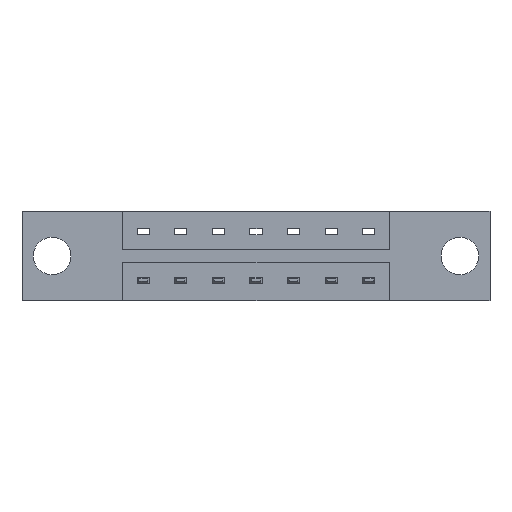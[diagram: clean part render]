
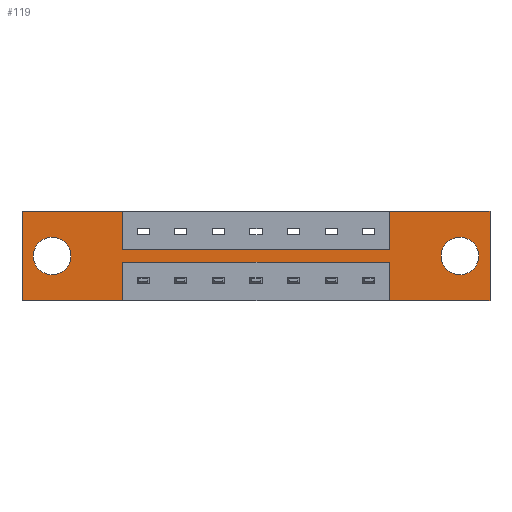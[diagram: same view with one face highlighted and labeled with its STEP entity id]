
A CAD part, front view. The second image highlights one B-rep face of the part: STEP entity #119.
In plain terms, the highlighted planar face has unit normal (0, -1, 0).
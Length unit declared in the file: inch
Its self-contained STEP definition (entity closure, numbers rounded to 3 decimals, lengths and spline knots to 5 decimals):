
#56 = EDGE_CURVE ( 'NONE', #5576, #5710, #2943, .T. ) ;
#72 = AXIS2_PLACEMENT_3D ( 'NONE', #1393, #3893, #1264 ) ;
#119 = ADVANCED_FACE ( 'NONE', ( #5658, #4258, #1630 ), #8319, .T. ) ;
#120 = EDGE_CURVE ( 'NONE', #6968, #8286, #5614, .T. ) ;
#171 = ORIENTED_EDGE ( 'NONE', *, *, #4753, .F. ) ;
#228 = LINE ( 'NONE', #2906, #4995 ) ;
#235 = ORIENTED_EDGE ( 'NONE', *, *, #6564, .F. ) ;
#274 = LINE ( 'NONE', #7508, #5452 ) ;
#319 = VERTEX_POINT ( 'NONE', #5963 ) ;
#415 = LINE ( 'NONE', #5751, #2326 ) ;
#420 = ORIENTED_EDGE ( 'NONE', *, *, #2875, .F. ) ;
#724 = CARTESIAN_POINT ( 'NONE',  ( 0.125, 0., -0.185 ) ) ;
#770 = ORIENTED_EDGE ( 'NONE', *, *, #2677, .F. ) ;
#819 = ORIENTED_EDGE ( 'NONE', *, *, #1943, .F. ) ;
#827 = ORIENTED_EDGE ( 'NONE', *, *, #1180, .F. ) ;
#941 = LINE ( 'NONE', #3728, #6771 ) ;
#965 = VERTEX_POINT ( 'NONE', #3575 ) ;
#981 = CARTESIAN_POINT ( 'NONE',  ( 0.4175, 0., -0.1585 ) ) ;
#1003 = VERTEX_POINT ( 'NONE', #1655 ) ;
#1050 = DIRECTION ( 'NONE',  ( 0., 0., -1. ) ) ;
#1118 = CARTESIAN_POINT ( 'NONE',  ( 0.4175, 0., -0.2115 ) ) ;
#1180 = EDGE_CURVE ( 'NONE', #1003, #2421, #8031, .T. ) ;
#1247 = DIRECTION ( 'NONE',  ( 1., 0., 0. ) ) ;
#1264 = DIRECTION ( 'NONE',  ( 0., 0., 1. ) ) ;
#1393 = CARTESIAN_POINT ( 'NONE',  ( 0.125, 0., -0.185 ) ) ;
#1422 = EDGE_CURVE ( 'NONE', #965, #4962, #941, .T. ) ;
#1538 = CARTESIAN_POINT ( 'NONE',  ( 0., 0., -0.37 ) ) ;
#1548 = VECTOR ( 'NONE', #3085, 39.37008 ) ;
#1630 = FACE_OUTER_BOUND ( 'NONE', #1774, .T. ) ;
#1648 = CARTESIAN_POINT ( 'NONE',  ( 0.4175, 0., -0.2115 ) ) ;
#1655 = CARTESIAN_POINT ( 'NONE',  ( 0., 0., 0. ) ) ;
#1774 = EDGE_LOOP ( 'NONE', ( #2347, #4719, #420, #2455, #770, #3944, #171, #827, #235, #4479, #4236, #819 ) ) ;
#1817 = DIRECTION ( 'NONE',  ( -1., 0., 0. ) ) ;
#1943 = EDGE_CURVE ( 'NONE', #4962, #7129, #228, .T. ) ;
#2043 = VERTEX_POINT ( 'NONE', #3120 ) ;
#2137 = EDGE_CURVE ( 'NONE', #2043, #2488, #8067, .T. ) ;
#2326 = VECTOR ( 'NONE', #3871, 39.37008 ) ;
#2347 = ORIENTED_EDGE ( 'NONE', *, *, #1422, .F. ) ;
#2374 = DIRECTION ( 'NONE',  ( 0., 0., 1. ) ) ;
#2390 = DIRECTION ( 'NONE',  ( 0., 0., -1. ) ) ;
#2394 = VERTEX_POINT ( 'NONE', #3150 ) ;
#2421 = VERTEX_POINT ( 'NONE', #3197 ) ;
#2455 = ORIENTED_EDGE ( 'NONE', *, *, #2630, .F. ) ;
#2488 = VERTEX_POINT ( 'NONE', #2498 ) ;
#2491 = LINE ( 'NONE', #1648, #8175 ) ;
#2498 = CARTESIAN_POINT ( 'NONE',  ( 1.815, 0., -0.263 ) ) ;
#2586 = CIRCLE ( 'NONE', #3675, 0.078 ) ;
#2630 = EDGE_CURVE ( 'NONE', #8416, #3316, #6665, .T. ) ;
#2677 = EDGE_CURVE ( 'NONE', #8286, #8416, #4085, .T. ) ;
#2875 = EDGE_CURVE ( 'NONE', #3316, #319, #274, .T. ) ;
#2906 = CARTESIAN_POINT ( 'NONE',  ( 0.4175, 0., -0.2115 ) ) ;
#2943 = CIRCLE ( 'NONE', #7828, 0.078 ) ;
#3085 = DIRECTION ( 'NONE',  ( 1., 0., 0. ) ) ;
#3120 = CARTESIAN_POINT ( 'NONE',  ( 1.815, 0., -0.107 ) ) ;
#3150 = CARTESIAN_POINT ( 'NONE',  ( 0.4175, 0., -0.37 ) ) ;
#3197 = CARTESIAN_POINT ( 'NONE',  ( 0.4175, 0., 0. ) ) ;
#3316 = VERTEX_POINT ( 'NONE', #3619 ) ;
#3478 = DIRECTION ( 'NONE',  ( 0., 1., 0. ) ) ;
#3533 = DIRECTION ( 'NONE',  ( 0., 0., -1. ) ) ;
#3575 = CARTESIAN_POINT ( 'NONE',  ( 1.5225, 0., -0.37 ) ) ;
#3594 = VECTOR ( 'NONE', #6621, 39.37008 ) ;
#3619 = CARTESIAN_POINT ( 'NONE',  ( 1.94, 0., 0. ) ) ;
#3675 = AXIS2_PLACEMENT_3D ( 'NONE', #7534, #5475, #3533 ) ;
#3728 = CARTESIAN_POINT ( 'NONE',  ( 1.5225, 0., -0.2115 ) ) ;
#3871 = DIRECTION ( 'NONE',  ( 0., 0., 1. ) ) ;
#3874 = AXIS2_PLACEMENT_3D ( 'NONE', #4076, #6699, #6826 ) ;
#3893 = DIRECTION ( 'NONE',  ( 0., 1., 0. ) ) ;
#3944 = ORIENTED_EDGE ( 'NONE', *, *, #120, .F. ) ;
#4076 = CARTESIAN_POINT ( 'NONE',  ( 1.815, 0., -0.185 ) ) ;
#4085 = LINE ( 'NONE', #6580, #3594 ) ;
#4092 = CARTESIAN_POINT ( 'NONE',  ( 0., 0., 0. ) ) ;
#4102 = EDGE_CURVE ( 'NONE', #2394, #4304, #7671, .T. ) ;
#4175 = DIRECTION ( 'NONE',  ( 0., 0., -1. ) ) ;
#4236 = ORIENTED_EDGE ( 'NONE', *, *, #5077, .F. ) ;
#4251 = DIRECTION ( 'NONE',  ( -1., 0., 0. ) ) ;
#4258 = FACE_BOUND ( 'NONE', #6367, .T. ) ;
#4304 = VERTEX_POINT ( 'NONE', #4520 ) ;
#4370 = CARTESIAN_POINT ( 'NONE',  ( 0.4175, 0., -0.1585 ) ) ;
#4452 = VECTOR ( 'NONE', #4251, 39.37008 ) ;
#4479 = ORIENTED_EDGE ( 'NONE', *, *, #4102, .F. ) ;
#4520 = CARTESIAN_POINT ( 'NONE',  ( 0., 0., -0.37 ) ) ;
#4583 = CARTESIAN_POINT ( 'NONE',  ( 0., 0., -0.37 ) ) ;
#4719 = ORIENTED_EDGE ( 'NONE', *, *, #7145, .F. ) ;
#4753 = EDGE_CURVE ( 'NONE', #2421, #6968, #8431, .T. ) ;
#4870 = EDGE_CURVE ( 'NONE', #5710, #5576, #5805, .T. ) ;
#4927 = ORIENTED_EDGE ( 'NONE', *, *, #56, .T. ) ;
#4962 = VERTEX_POINT ( 'NONE', #6770 ) ;
#4995 = VECTOR ( 'NONE', #5572, 39.37008 ) ;
#5077 = EDGE_CURVE ( 'NONE', #7129, #2394, #2491, .T. ) ;
#5161 = CARTESIAN_POINT ( 'NONE',  ( 1.5225, 0., 0. ) ) ;
#5278 = CARTESIAN_POINT ( 'NONE',  ( 0., 0., 0. ) ) ;
#5452 = VECTOR ( 'NONE', #4175, 39.37008 ) ;
#5475 = DIRECTION ( 'NONE',  ( 0., 1., 0. ) ) ;
#5572 = DIRECTION ( 'NONE',  ( -1., 0., 0. ) ) ;
#5576 = VERTEX_POINT ( 'NONE', #7681 ) ;
#5614 = LINE ( 'NONE', #981, #1548 ) ;
#5658 = FACE_BOUND ( 'NONE', #6966, .T. ) ;
#5710 = VERTEX_POINT ( 'NONE', #6489 ) ;
#5751 = CARTESIAN_POINT ( 'NONE',  ( 0., 0., 0. ) ) ;
#5805 = CIRCLE ( 'NONE', #72, 0.078 ) ;
#5844 = VECTOR ( 'NONE', #1247, 39.37008 ) ;
#5963 = CARTESIAN_POINT ( 'NONE',  ( 1.94, 0., -0.37 ) ) ;
#6058 = DIRECTION ( 'NONE',  ( 0., 0., 1. ) ) ;
#6061 = ORIENTED_EDGE ( 'NONE', *, *, #2137, .T. ) ;
#6166 = CARTESIAN_POINT ( 'NONE',  ( 1.5225, 0., -0.1585 ) ) ;
#6367 = EDGE_LOOP ( 'NONE', ( #8427, #4927 ) ) ;
#6394 = CARTESIAN_POINT ( 'NONE',  ( 0., 0., -0.37 ) ) ;
#6429 = AXIS2_PLACEMENT_3D ( 'NONE', #6394, #7011, #8403 ) ;
#6489 = CARTESIAN_POINT ( 'NONE',  ( 0.125, 0., -0.107 ) ) ;
#6493 = LINE ( 'NONE', #4583, #8615 ) ;
#6564 = EDGE_CURVE ( 'NONE', #4304, #1003, #415, .T. ) ;
#6580 = CARTESIAN_POINT ( 'NONE',  ( 1.5225, 0., -0.1585 ) ) ;
#6621 = DIRECTION ( 'NONE',  ( 0., 0., 1. ) ) ;
#6665 = LINE ( 'NONE', #5278, #5844 ) ;
#6699 = DIRECTION ( 'NONE',  ( 0., 1., 0. ) ) ;
#6770 = CARTESIAN_POINT ( 'NONE',  ( 1.5225, 0., -0.2115 ) ) ;
#6771 = VECTOR ( 'NONE', #2374, 39.37008 ) ;
#6826 = DIRECTION ( 'NONE',  ( 0., 0., -1. ) ) ;
#6844 = DIRECTION ( 'NONE',  ( 1., 0., 0. ) ) ;
#6966 = EDGE_LOOP ( 'NONE', ( #6061, #7082 ) ) ;
#6968 = VERTEX_POINT ( 'NONE', #7018 ) ;
#7011 = DIRECTION ( 'NONE',  ( 0., -1., 0. ) ) ;
#7018 = CARTESIAN_POINT ( 'NONE',  ( 0.4175, 0., -0.1585 ) ) ;
#7028 = VECTOR ( 'NONE', #6844, 39.37008 ) ;
#7082 = ORIENTED_EDGE ( 'NONE', *, *, #8332, .T. ) ;
#7129 = VERTEX_POINT ( 'NONE', #1118 ) ;
#7145 = EDGE_CURVE ( 'NONE', #319, #965, #6493, .T. ) ;
#7463 = VECTOR ( 'NONE', #1050, 39.37008 ) ;
#7508 = CARTESIAN_POINT ( 'NONE',  ( 1.94, 0., 0. ) ) ;
#7534 = CARTESIAN_POINT ( 'NONE',  ( 1.815, 0., -0.185 ) ) ;
#7671 = LINE ( 'NONE', #1538, #4452 ) ;
#7681 = CARTESIAN_POINT ( 'NONE',  ( 0.125, 0., -0.263 ) ) ;
#7828 = AXIS2_PLACEMENT_3D ( 'NONE', #724, #3478, #6058 ) ;
#8031 = LINE ( 'NONE', #4092, #7028 ) ;
#8067 = CIRCLE ( 'NONE', #3874, 0.078 ) ;
#8175 = VECTOR ( 'NONE', #2390, 39.37008 ) ;
#8286 = VERTEX_POINT ( 'NONE', #6166 ) ;
#8319 = PLANE ( 'NONE',  #6429 ) ;
#8332 = EDGE_CURVE ( 'NONE', #2488, #2043, #2586, .T. ) ;
#8403 = DIRECTION ( 'NONE',  ( 0., 0., -1. ) ) ;
#8416 = VERTEX_POINT ( 'NONE', #5161 ) ;
#8427 = ORIENTED_EDGE ( 'NONE', *, *, #4870, .T. ) ;
#8431 = LINE ( 'NONE', #4370, #7463 ) ;
#8615 = VECTOR ( 'NONE', #1817, 39.37008 ) ;
